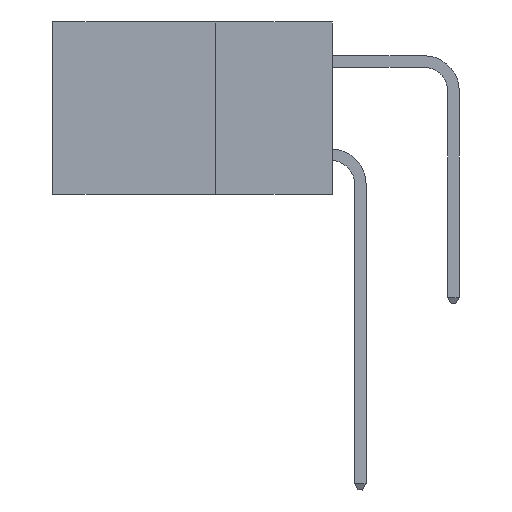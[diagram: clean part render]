
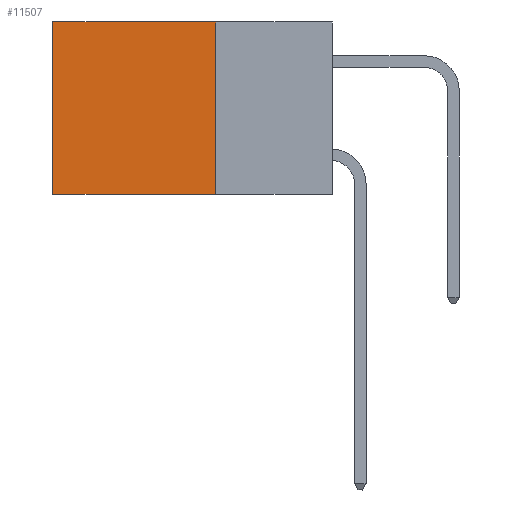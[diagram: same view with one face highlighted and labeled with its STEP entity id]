
A CAD part, left-side view. The second image highlights one B-rep face of the part: STEP entity #11507.
In plain terms, the highlighted planar face has unit normal (-1, 0, 0).
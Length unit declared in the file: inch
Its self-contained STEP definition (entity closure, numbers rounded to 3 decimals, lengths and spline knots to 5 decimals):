
#172 = LINE ( 'NONE', #1395, #285 ) ;
#285 = VECTOR ( 'NONE', #10862, 39.37008 ) ;
#1395 = CARTESIAN_POINT ( 'NONE',  ( 0.2615, 0.25, 0. ) ) ;
#1679 = CARTESIAN_POINT ( 'NONE',  ( 0.2615, 0.6, 0. ) ) ;
#1681 = ORIENTED_EDGE ( 'NONE', *, *, #5503, .F. ) ;
#1795 = FACE_OUTER_BOUND ( 'NONE', #11769, .T. ) ;
#2480 = CARTESIAN_POINT ( 'NONE',  ( 0.2615, 0.25, -0.37 ) ) ;
#2498 = CARTESIAN_POINT ( 'NONE',  ( 0.2615, 0.25, 0. ) ) ;
#2649 = CARTESIAN_POINT ( 'NONE',  ( 0.2615, 0.25, -0.37 ) ) ;
#3282 = ORIENTED_EDGE ( 'NONE', *, *, #13486, .T. ) ;
#3756 = LINE ( 'NONE', #2480, #9526 ) ;
#4193 = CARTESIAN_POINT ( 'NONE',  ( 0.2615, 0.6, -0.37 ) ) ;
#5503 = EDGE_CURVE ( 'NONE', #7698, #9528, #3756, .T. ) ;
#6005 = CARTESIAN_POINT ( 'NONE',  ( 0.2615, 0.6, -0.37 ) ) ;
#6097 = DIRECTION ( 'NONE',  ( 1., 0., 0. ) ) ;
#6556 = VERTEX_POINT ( 'NONE', #1679 ) ;
#6709 = DIRECTION ( 'NONE',  ( 0., 1., 0. ) ) ;
#6727 = VECTOR ( 'NONE', #12628, 39.37008 ) ;
#6783 = EDGE_CURVE ( 'NONE', #7738, #6556, #172, .T. ) ;
#7031 = EDGE_CURVE ( 'NONE', #7738, #7698, #12868, .T. ) ;
#7525 = DIRECTION ( 'NONE',  ( 0., 0., -1. ) ) ;
#7698 = VERTEX_POINT ( 'NONE', #9767 ) ;
#7738 = VERTEX_POINT ( 'NONE', #2498 ) ;
#8289 = PLANE ( 'NONE',  #12287 ) ;
#8884 = ORIENTED_EDGE ( 'NONE', *, *, #6783, .T. ) ;
#9149 = DIRECTION ( 'NONE',  ( 0., 0., -1. ) ) ;
#9407 = LINE ( 'NONE', #4193, #6727 ) ;
#9526 = VECTOR ( 'NONE', #6709, 39.37008 ) ;
#9528 = VERTEX_POINT ( 'NONE', #6005 ) ;
#9649 = CARTESIAN_POINT ( 'NONE',  ( 0.2615, 0.25, -0.37 ) ) ;
#9767 = CARTESIAN_POINT ( 'NONE',  ( 0.2615, 0.25, -0.37 ) ) ;
#10024 = VECTOR ( 'NONE', #7525, 39.37008 ) ;
#10862 = DIRECTION ( 'NONE',  ( 0., 1., 0. ) ) ;
#11507 = ADVANCED_FACE ( 'NONE', ( #1795 ), #8289, .F. ) ;
#11769 = EDGE_LOOP ( 'NONE', ( #3282, #1681, #12196, #8884 ) ) ;
#12196 = ORIENTED_EDGE ( 'NONE', *, *, #7031, .F. ) ;
#12287 = AXIS2_PLACEMENT_3D ( 'NONE', #2649, #6097, #9149 ) ;
#12628 = DIRECTION ( 'NONE',  ( 0., 0., -1. ) ) ;
#12868 = LINE ( 'NONE', #9649, #10024 ) ;
#13486 = EDGE_CURVE ( 'NONE', #6556, #9528, #9407, .T. ) ;
